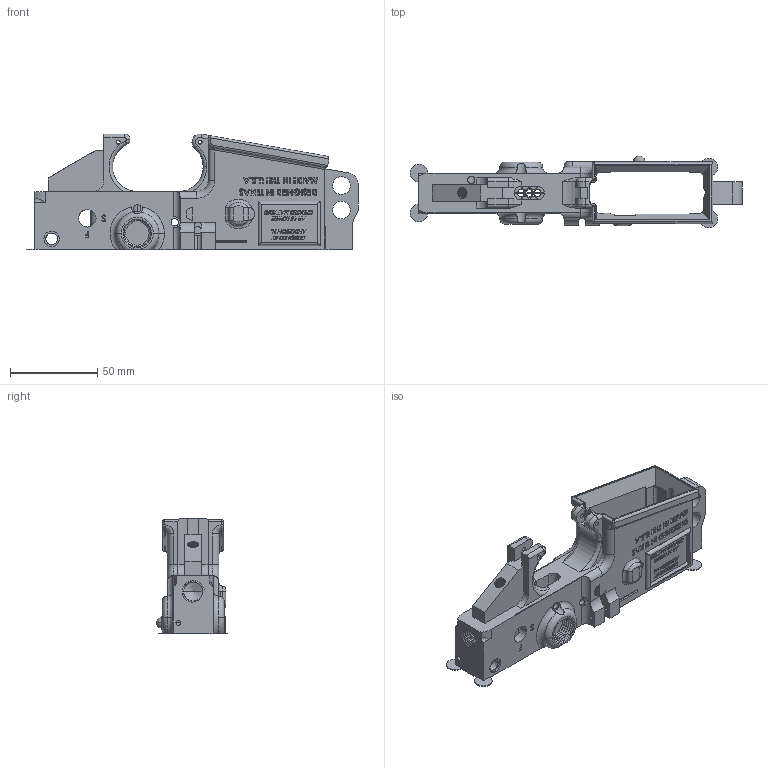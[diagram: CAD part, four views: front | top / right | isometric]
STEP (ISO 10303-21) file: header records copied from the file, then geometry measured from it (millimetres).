
FILE_DESCRIPTION (( 'STEP AP203' ), '1' );
FILE_NAME ('AF-WF-LR-PRT-001-SLDWRKS.STEP', '2020-07-21T18:13:39', ( '' ), ( '' ), 'SwSTEP 2.0', 'SolidWorks 2018', '' );
FILE_SCHEMA (( 'CONFIG_CONTROL_DESIGN' ));
Length unit declared in the file: inch
Products named in the file (1): AF-WF-LR-PRT-001-SLDWRKS
Bounding box: 189.94 x 41.05 x 66.36 mm (x, y, z)
Volume: 86129.7 mm3; surface area: 65087.7 mm2
Topology: 1 solids, 13 shells, 2517 faces, 6965 edges, 4610 vertices
Faces by surface type: plane 1614, bspline 578, cylinder 282, torus 31, sphere 6, cone 6
Entity records: 123922 total; most frequent: CARTESIAN_POINT 64061, ORIENTED_EDGE 13906, DIRECTION 9837, EDGE_CURVE 6953, LINE 4917, VECTOR 4917, VERTEX_POINT 4606, EDGE_LOOP 2729
